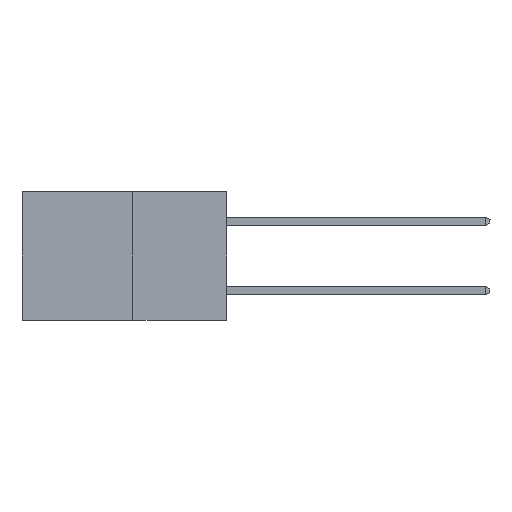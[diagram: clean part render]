
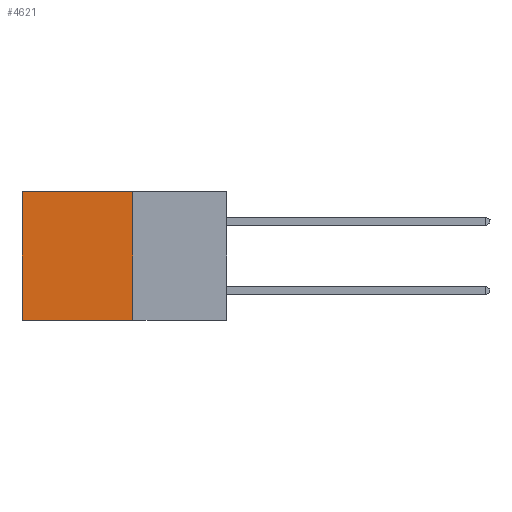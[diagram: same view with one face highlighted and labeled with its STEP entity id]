
A CAD part, left-side view. The second image highlights one B-rep face of the part: STEP entity #4621.
In plain terms, the highlighted planar face has unit normal (-1, 0, 0).
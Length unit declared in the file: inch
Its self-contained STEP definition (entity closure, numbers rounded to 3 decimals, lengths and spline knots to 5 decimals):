
#180 = CARTESIAN_POINT ( 'NONE',  ( 0.277, 0.27, -0.37 ) ) ;
#1815 = CARTESIAN_POINT ( 'NONE',  ( 0.277, 0.27, -0.37 ) ) ;
#1912 = VERTEX_POINT ( 'NONE', #8607 ) ;
#2140 = DIRECTION ( 'NONE',  ( 0., 1., 0. ) ) ;
#2425 = DIRECTION ( 'NONE',  ( 1., 0., 0. ) ) ;
#2565 = LINE ( 'NONE', #180, #14946 ) ;
#2793 = EDGE_CURVE ( 'NONE', #1912, #12364, #2565, .T. ) ;
#2806 = LINE ( 'NONE', #14365, #9772 ) ;
#3185 = FACE_OUTER_BOUND ( 'NONE', #4254, .T. ) ;
#3582 = VERTEX_POINT ( 'NONE', #15051 ) ;
#3702 = VERTEX_POINT ( 'NONE', #18172 ) ;
#4067 = EDGE_CURVE ( 'NONE', #3702, #1912, #7301, .T. ) ;
#4254 = EDGE_LOOP ( 'NONE', ( #10204, #10636, #15381, #16221 ) ) ;
#4271 = PLANE ( 'NONE',  #12514 ) ;
#4621 = ADVANCED_FACE ( 'NONE', ( #3185 ), #4271, .F. ) ;
#5845 = DIRECTION ( 'NONE',  ( 0., 0., -1. ) ) ;
#7301 = LINE ( 'NONE', #16571, #10925 ) ;
#8607 = CARTESIAN_POINT ( 'NONE',  ( 0.277, 0.27, -0.37 ) ) ;
#8708 = CARTESIAN_POINT ( 'NONE',  ( 0.277, 0.59, -0.37 ) ) ;
#9772 = VECTOR ( 'NONE', #12254, 39.37008 ) ;
#10204 = ORIENTED_EDGE ( 'NONE', *, *, #11432, .T. ) ;
#10636 = ORIENTED_EDGE ( 'NONE', *, *, #2793, .F. ) ;
#10925 = VECTOR ( 'NONE', #17493, 39.37008 ) ;
#11017 = DIRECTION ( 'NONE',  ( 0., 1., 0. ) ) ;
#11432 = EDGE_CURVE ( 'NONE', #3582, #12364, #2806, .T. ) ;
#12204 = LINE ( 'NONE', #16009, #19697 ) ;
#12254 = DIRECTION ( 'NONE',  ( 0., 0., -1. ) ) ;
#12364 = VERTEX_POINT ( 'NONE', #8708 ) ;
#12514 = AXIS2_PLACEMENT_3D ( 'NONE', #1815, #2425, #5845 ) ;
#14365 = CARTESIAN_POINT ( 'NONE',  ( 0.277, 0.59, -0.37 ) ) ;
#14946 = VECTOR ( 'NONE', #11017, 39.37008 ) ;
#15051 = CARTESIAN_POINT ( 'NONE',  ( 0.277, 0.59, 0. ) ) ;
#15381 = ORIENTED_EDGE ( 'NONE', *, *, #4067, .F. ) ;
#16009 = CARTESIAN_POINT ( 'NONE',  ( 0.277, 0.27, 0. ) ) ;
#16221 = ORIENTED_EDGE ( 'NONE', *, *, #18332, .T. ) ;
#16571 = CARTESIAN_POINT ( 'NONE',  ( 0.277, 0.27, -0.37 ) ) ;
#17493 = DIRECTION ( 'NONE',  ( 0., 0., -1. ) ) ;
#18172 = CARTESIAN_POINT ( 'NONE',  ( 0.277, 0.27, 0. ) ) ;
#18332 = EDGE_CURVE ( 'NONE', #3702, #3582, #12204, .T. ) ;
#19697 = VECTOR ( 'NONE', #2140, 39.37008 ) ;
